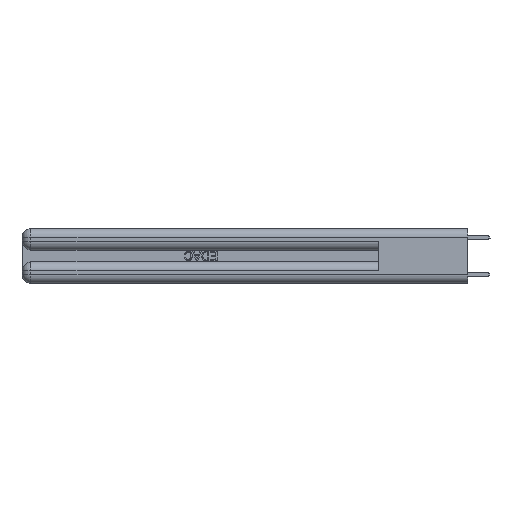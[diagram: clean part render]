
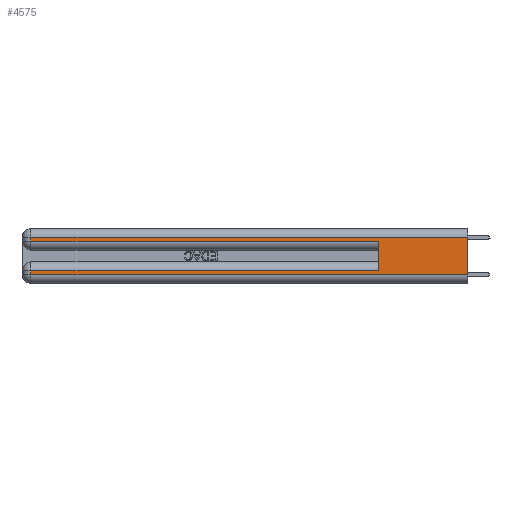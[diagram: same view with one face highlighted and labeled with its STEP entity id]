
A CAD part, left-side view. The second image highlights one B-rep face of the part: STEP entity #4575.
In plain terms, the highlighted planar face has unit normal (-1, 0, 0).
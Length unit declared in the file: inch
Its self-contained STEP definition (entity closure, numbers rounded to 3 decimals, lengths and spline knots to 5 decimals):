
#41 = VERTEX_POINT ( 'NONE', #14196 ) ;
#586 = VERTEX_POINT ( 'NONE', #19235 ) ;
#811 = EDGE_CURVE ( 'NONE', #11032, #27186, #16399, .T. ) ;
#1289 = VECTOR ( 'NONE', #2557, 39.37008 ) ;
#1705 = LINE ( 'NONE', #23909, #17445 ) ;
#2058 = VERTEX_POINT ( 'NONE', #19152 ) ;
#2119 = DIRECTION ( 'NONE',  ( 0., 1., 0. ) ) ;
#2529 = VECTOR ( 'NONE', #14934, 39.37008 ) ;
#2557 = DIRECTION ( 'NONE',  ( 0., 0., -1. ) ) ;
#3080 = VERTEX_POINT ( 'NONE', #24422 ) ;
#3543 = DIRECTION ( 'NONE',  ( 0., 1., 0. ) ) ;
#4575 = ADVANCED_FACE ( 'NONE', ( #10403 ), #6640, .F. ) ;
#4861 = ORIENTED_EDGE ( 'NONE', *, *, #9812, .T. ) ;
#4940 = VERTEX_POINT ( 'NONE', #7713 ) ;
#5265 = EDGE_CURVE ( 'NONE', #29512, #2058, #15470, .T. ) ;
#6079 = DIRECTION ( 'NONE',  ( 0., -1., 0. ) ) ;
#6145 = CARTESIAN_POINT ( 'NONE',  ( 0., 0.6, 0.085 ) ) ;
#6268 = LINE ( 'NONE', #29765, #31137 ) ;
#6455 = EDGE_CURVE ( 'NONE', #41, #4940, #21363, .T. ) ;
#6640 = PLANE ( 'NONE',  #23963 ) ;
#7591 = CARTESIAN_POINT ( 'NONE',  ( 0., 2.94, 0.37 ) ) ;
#7713 = CARTESIAN_POINT ( 'NONE',  ( 0., 2.94, 0.285 ) ) ;
#7732 = LINE ( 'NONE', #12544, #17578 ) ;
#8363 = CARTESIAN_POINT ( 'NONE',  ( 0., 0., 0.085 ) ) ;
#9261 = CARTESIAN_POINT ( 'NONE',  ( 0., 0., 0.37 ) ) ;
#9581 = CARTESIAN_POINT ( 'NONE',  ( 0., 0., 0.06 ) ) ;
#9812 = EDGE_CURVE ( 'NONE', #11032, #41, #6268, .T. ) ;
#10140 = LINE ( 'NONE', #8363, #30275 ) ;
#10403 = FACE_OUTER_BOUND ( 'NONE', #27047, .T. ) ;
#11032 = VERTEX_POINT ( 'NONE', #30668 ) ;
#11374 = CARTESIAN_POINT ( 'NONE',  ( 0., 0., 0.285 ) ) ;
#11557 = CARTESIAN_POINT ( 'NONE',  ( 0., 0., 0.37 ) ) ;
#12544 = CARTESIAN_POINT ( 'NONE',  ( 0., 2.94, 0.37 ) ) ;
#13701 = DIRECTION ( 'NONE',  ( 0., -1., 0. ) ) ;
#14196 = CARTESIAN_POINT ( 'NONE',  ( 0., 2.94, 0.31 ) ) ;
#14444 = ORIENTED_EDGE ( 'NONE', *, *, #20568, .T. ) ;
#14934 = DIRECTION ( 'NONE',  ( 0., 0., 1. ) ) ;
#15470 = LINE ( 'NONE', #28497, #2529 ) ;
#16078 = ORIENTED_EDGE ( 'NONE', *, *, #6455, .T. ) ;
#16399 = LINE ( 'NONE', #9261, #29825 ) ;
#16591 = ORIENTED_EDGE ( 'NONE', *, *, #22064, .T. ) ;
#17445 = VECTOR ( 'NONE', #6079, 39.37008 ) ;
#17578 = VECTOR ( 'NONE', #30225, 39.37008 ) ;
#18443 = ORIENTED_EDGE ( 'NONE', *, *, #27736, .T. ) ;
#19152 = CARTESIAN_POINT ( 'NONE',  ( 0., 0.6, 0.285 ) ) ;
#19235 = CARTESIAN_POINT ( 'NONE',  ( 0., 2.94, 0.085 ) ) ;
#20568 = EDGE_CURVE ( 'NONE', #3080, #27186, #1705, .T. ) ;
#21363 = LINE ( 'NONE', #7591, #1289 ) ;
#22064 = EDGE_CURVE ( 'NONE', #586, #3080, #7732, .T. ) ;
#23841 = DIRECTION ( 'NONE',  ( 1., 0., 0. ) ) ;
#23909 = CARTESIAN_POINT ( 'NONE',  ( 0., 0., 0.06 ) ) ;
#23963 = AXIS2_PLACEMENT_3D ( 'NONE', #11557, #23841, #24174 ) ;
#24174 = DIRECTION ( 'NONE',  ( 0., 0., -1. ) ) ;
#24422 = CARTESIAN_POINT ( 'NONE',  ( 0., 2.94, 0.06 ) ) ;
#24822 = EDGE_CURVE ( 'NONE', #4940, #2058, #31240, .T. ) ;
#25284 = ORIENTED_EDGE ( 'NONE', *, *, #811, .F. ) ;
#25696 = ORIENTED_EDGE ( 'NONE', *, *, #5265, .F. ) ;
#27047 = EDGE_LOOP ( 'NONE', ( #25284, #4861, #16078, #27629, #25696, #18443, #16591, #14444 ) ) ;
#27186 = VERTEX_POINT ( 'NONE', #9581 ) ;
#27287 = VECTOR ( 'NONE', #13701, 39.37008 ) ;
#27629 = ORIENTED_EDGE ( 'NONE', *, *, #24822, .T. ) ;
#27736 = EDGE_CURVE ( 'NONE', #29512, #586, #10140, .T. ) ;
#28497 = CARTESIAN_POINT ( 'NONE',  ( 0., 0.6, 0.145 ) ) ;
#29512 = VERTEX_POINT ( 'NONE', #6145 ) ;
#29765 = CARTESIAN_POINT ( 'NONE',  ( 0., 0., 0.31 ) ) ;
#29825 = VECTOR ( 'NONE', #32493, 39.37008 ) ;
#30225 = DIRECTION ( 'NONE',  ( 0., 0., -1. ) ) ;
#30275 = VECTOR ( 'NONE', #3543, 39.37008 ) ;
#30668 = CARTESIAN_POINT ( 'NONE',  ( 0., 0., 0.31 ) ) ;
#31137 = VECTOR ( 'NONE', #2119, 39.37008 ) ;
#31240 = LINE ( 'NONE', #11374, #27287 ) ;
#32493 = DIRECTION ( 'NONE',  ( 0., 0., -1. ) ) ;
